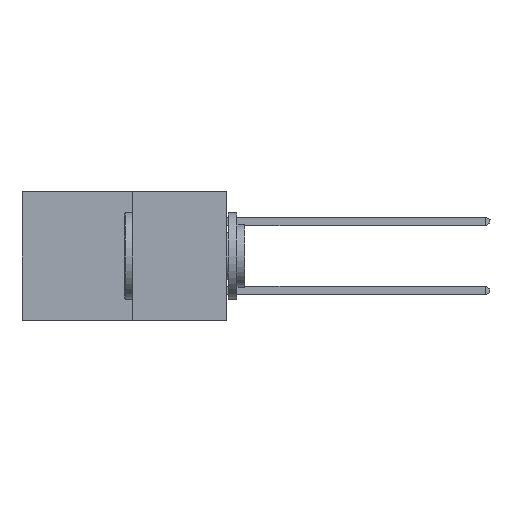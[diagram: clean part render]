
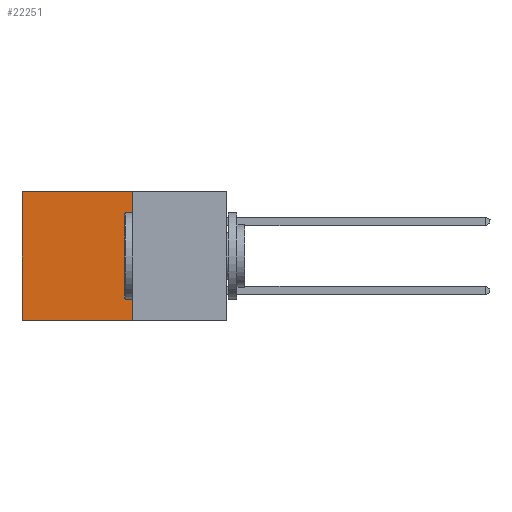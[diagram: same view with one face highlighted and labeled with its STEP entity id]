
A CAD part, left-side view. The second image highlights one B-rep face of the part: STEP entity #22251.
In plain terms, the highlighted planar face has unit normal (-1, 0, 0).
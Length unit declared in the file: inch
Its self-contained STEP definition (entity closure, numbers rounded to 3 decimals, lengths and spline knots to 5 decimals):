
#1106 = LINE ( 'NONE', #29915, #12237 ) ;
#1885 = DIRECTION ( 'NONE',  ( 0., 0., -1. ) ) ;
#2530 = DIRECTION ( 'NONE',  ( 0., 1., 0. ) ) ;
#2595 = DIRECTION ( 'NONE',  ( 0., 0., -1. ) ) ;
#2716 = CARTESIAN_POINT ( 'NONE',  ( 0.277, 0.27, -0.37 ) ) ;
#5151 = AXIS2_PLACEMENT_3D ( 'NONE', #14423, #16786, #2595 ) ;
#6241 = VERTEX_POINT ( 'NONE', #2716 ) ;
#7357 = VERTEX_POINT ( 'NONE', #25922 ) ;
#7379 = DIRECTION ( 'NONE',  ( 0., 1., 0. ) ) ;
#8522 = LINE ( 'NONE', #25464, #21115 ) ;
#8623 = VERTEX_POINT ( 'NONE', #25357 ) ;
#8745 = DIRECTION ( 'NONE',  ( 0., 0., -1. ) ) ;
#8872 = LINE ( 'NONE', #9773, #21145 ) ;
#8902 = EDGE_CURVE ( 'NONE', #6241, #8623, #8872, .T. ) ;
#9388 = EDGE_CURVE ( 'NONE', #17362, #6241, #8522, .T. ) ;
#9592 = CARTESIAN_POINT ( 'NONE',  ( 0.277, 0.27, 0. ) ) ;
#9773 = CARTESIAN_POINT ( 'NONE',  ( 0.277, 0.27, -0.37 ) ) ;
#10069 = ORIENTED_EDGE ( 'NONE', *, *, #19884, .T. ) ;
#12237 = VECTOR ( 'NONE', #8745, 39.37008 ) ;
#13800 = ORIENTED_EDGE ( 'NONE', *, *, #9388, .F. ) ;
#14423 = CARTESIAN_POINT ( 'NONE',  ( 0.277, 0.27, -0.37 ) ) ;
#15925 = CARTESIAN_POINT ( 'NONE',  ( 0.277, 0.27, 0. ) ) ;
#16786 = DIRECTION ( 'NONE',  ( 1., 0., 0. ) ) ;
#17362 = VERTEX_POINT ( 'NONE', #15925 ) ;
#17785 = VECTOR ( 'NONE', #2530, 39.37008 ) ;
#19884 = EDGE_CURVE ( 'NONE', #17362, #7357, #30239, .T. ) ;
#20319 = EDGE_CURVE ( 'NONE', #7357, #8623, #1106, .T. ) ;
#20624 = FACE_OUTER_BOUND ( 'NONE', #25119, .T. ) ;
#21115 = VECTOR ( 'NONE', #1885, 39.37008 ) ;
#21145 = VECTOR ( 'NONE', #7379, 39.37008 ) ;
#22251 = ADVANCED_FACE ( 'NONE', ( #20624 ), #28488, .F. ) ;
#25119 = EDGE_LOOP ( 'NONE', ( #25742, #27641, #13800, #10069 ) ) ;
#25357 = CARTESIAN_POINT ( 'NONE',  ( 0.277, 0.59, -0.37 ) ) ;
#25464 = CARTESIAN_POINT ( 'NONE',  ( 0.277, 0.27, -0.37 ) ) ;
#25742 = ORIENTED_EDGE ( 'NONE', *, *, #20319, .T. ) ;
#25922 = CARTESIAN_POINT ( 'NONE',  ( 0.277, 0.59, 0. ) ) ;
#27641 = ORIENTED_EDGE ( 'NONE', *, *, #8902, .F. ) ;
#28488 = PLANE ( 'NONE',  #5151 ) ;
#29915 = CARTESIAN_POINT ( 'NONE',  ( 0.277, 0.59, -0.37 ) ) ;
#30239 = LINE ( 'NONE', #9592, #17785 ) ;
